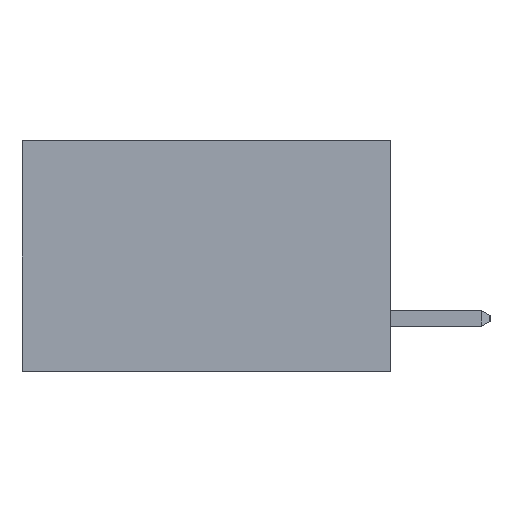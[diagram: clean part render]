
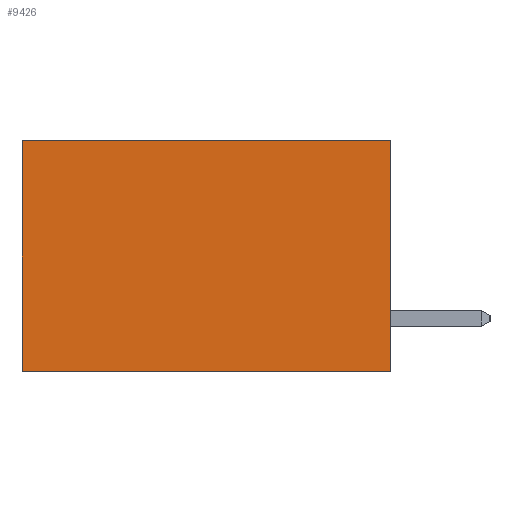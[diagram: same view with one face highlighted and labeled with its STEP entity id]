
A CAD part, left-side view. The second image highlights one B-rep face of the part: STEP entity #9426.
In plain terms, the highlighted planar face has unit normal (-1, 0, 0).
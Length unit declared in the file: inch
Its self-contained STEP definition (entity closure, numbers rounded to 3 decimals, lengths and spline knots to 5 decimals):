
#623 = CARTESIAN_POINT ( 'NONE',  ( 0.277, 0.59, 0. ) ) ;
#1021 = DIRECTION ( 'NONE',  ( 0., 0., -1. ) ) ;
#1511 = DIRECTION ( 'NONE',  ( 0., 0., -1. ) ) ;
#1627 = VECTOR ( 'NONE', #14918, 39.37008 ) ;
#5107 = EDGE_LOOP ( 'NONE', ( #20695, #12679, #7062, #25796 ) ) ;
#5507 = CARTESIAN_POINT ( 'NONE',  ( 0.277, 0., -0.37 ) ) ;
#6550 = VERTEX_POINT ( 'NONE', #11218 ) ;
#7043 = LINE ( 'NONE', #12885, #1627 ) ;
#7062 = ORIENTED_EDGE ( 'NONE', *, *, #19868, .F. ) ;
#7217 = DIRECTION ( 'NONE',  ( 0., 0., -1. ) ) ;
#7311 = LINE ( 'NONE', #11183, #12095 ) ;
#8394 = LINE ( 'NONE', #19414, #22674 ) ;
#9426 = ADVANCED_FACE ( 'NONE', ( #14440 ), #19791, .F. ) ;
#10788 = VERTEX_POINT ( 'NONE', #623 ) ;
#10805 = EDGE_CURVE ( 'NONE', #15603, #10788, #7043, .T. ) ;
#11183 = CARTESIAN_POINT ( 'NONE',  ( 0.277, 0.59, -0.37 ) ) ;
#11218 = CARTESIAN_POINT ( 'NONE',  ( 0.277, 0.59, -0.37 ) ) ;
#12095 = VECTOR ( 'NONE', #1021, 39.37008 ) ;
#12679 = ORIENTED_EDGE ( 'NONE', *, *, #16688, .F. ) ;
#12885 = CARTESIAN_POINT ( 'NONE',  ( 0.277, 0., 0. ) ) ;
#13403 = CARTESIAN_POINT ( 'NONE',  ( 0.277, 0., -0.37 ) ) ;
#13718 = DIRECTION ( 'NONE',  ( 1., 0., 0. ) ) ;
#14160 = CARTESIAN_POINT ( 'NONE',  ( 0.277, 0., -0.37 ) ) ;
#14435 = VERTEX_POINT ( 'NONE', #14160 ) ;
#14440 = FACE_OUTER_BOUND ( 'NONE', #5107, .T. ) ;
#14918 = DIRECTION ( 'NONE',  ( 0., 1., 0. ) ) ;
#15603 = VERTEX_POINT ( 'NONE', #20283 ) ;
#15943 = AXIS2_PLACEMENT_3D ( 'NONE', #5507, #13718, #1511 ) ;
#15984 = EDGE_CURVE ( 'NONE', #10788, #6550, #7311, .T. ) ;
#16688 = EDGE_CURVE ( 'NONE', #14435, #6550, #17133, .T. ) ;
#17133 = LINE ( 'NONE', #13403, #22540 ) ;
#19414 = CARTESIAN_POINT ( 'NONE',  ( 0.277, 0., -0.37 ) ) ;
#19791 = PLANE ( 'NONE',  #15943 ) ;
#19868 = EDGE_CURVE ( 'NONE', #15603, #14435, #8394, .T. ) ;
#20283 = CARTESIAN_POINT ( 'NONE',  ( 0.277, 0., 0. ) ) ;
#20695 = ORIENTED_EDGE ( 'NONE', *, *, #15984, .T. ) ;
#22540 = VECTOR ( 'NONE', #25507, 39.37008 ) ;
#22674 = VECTOR ( 'NONE', #7217, 39.37008 ) ;
#25507 = DIRECTION ( 'NONE',  ( 0., 1., 0. ) ) ;
#25796 = ORIENTED_EDGE ( 'NONE', *, *, #10805, .T. ) ;
